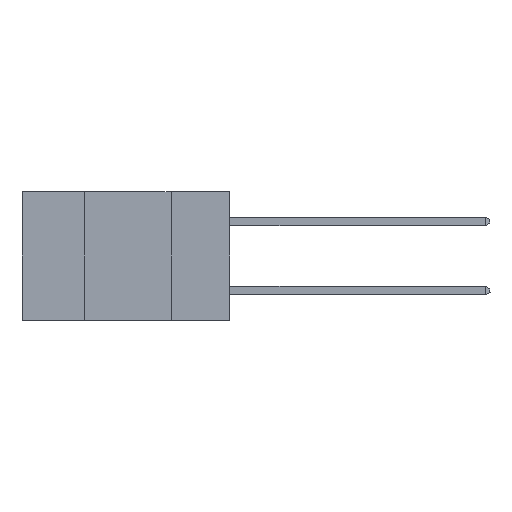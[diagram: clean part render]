
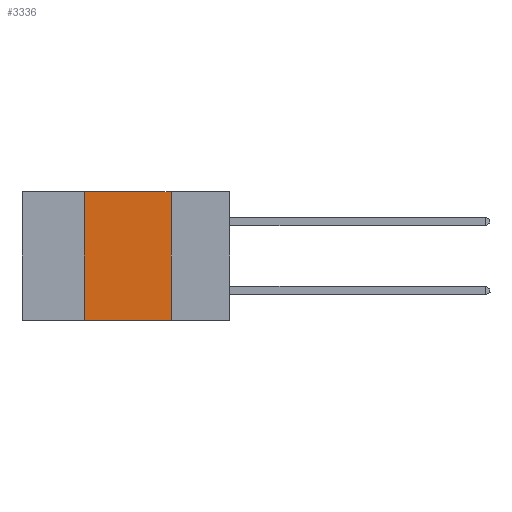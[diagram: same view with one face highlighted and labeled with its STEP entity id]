
A CAD part, left-side view. The second image highlights one B-rep face of the part: STEP entity #3336.
In plain terms, the highlighted planar face has unit normal (-1, 0, 0).
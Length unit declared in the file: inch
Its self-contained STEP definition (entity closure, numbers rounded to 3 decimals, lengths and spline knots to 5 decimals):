
#15 = EDGE_LOOP ( 'NONE', ( #10765, #5312, #13418, #7980 ) ) ;
#308 = FACE_OUTER_BOUND ( 'NONE', #15, .T. ) ;
#1269 = LINE ( 'NONE', #13963, #6182 ) ;
#1389 = CARTESIAN_POINT ( 'NONE',  ( 0., 0.6, 0. ) ) ;
#2230 = DIRECTION ( 'NONE',  ( 1., 0., 0. ) ) ;
#2913 = CARTESIAN_POINT ( 'NONE',  ( 0., 0.17, 0. ) ) ;
#3047 = CARTESIAN_POINT ( 'NONE',  ( 0., 0.17, 0. ) ) ;
#3236 = DIRECTION ( 'NONE',  ( 0., 0., 1. ) ) ;
#3336 = ADVANCED_FACE ( 'NONE', ( #308 ), #5546, .F. ) ;
#3437 = DIRECTION ( 'NONE',  ( 0., 0., -1. ) ) ;
#4242 = VERTEX_POINT ( 'NONE', #6245 ) ;
#4248 = EDGE_CURVE ( 'NONE', #11750, #12309, #8111, .T. ) ;
#4406 = LINE ( 'NONE', #2913, #5931 ) ;
#5312 = ORIENTED_EDGE ( 'NONE', *, *, #4248, .F. ) ;
#5546 = PLANE ( 'NONE',  #13192 ) ;
#5931 = VECTOR ( 'NONE', #11344, 39.37008 ) ;
#6182 = VECTOR ( 'NONE', #3236, 39.37008 ) ;
#6245 = CARTESIAN_POINT ( 'NONE',  ( 0., 0.17, -0.37 ) ) ;
#7114 = VECTOR ( 'NONE', #12608, 39.37008 ) ;
#7655 = CARTESIAN_POINT ( 'NONE',  ( 0., 0.42, -0.37 ) ) ;
#7980 = ORIENTED_EDGE ( 'NONE', *, *, #11260, .T. ) ;
#8111 = LINE ( 'NONE', #1389, #10176 ) ;
#8279 = LINE ( 'NONE', #12201, #7114 ) ;
#10176 = VECTOR ( 'NONE', #14512, 39.37008 ) ;
#10275 = CARTESIAN_POINT ( 'NONE',  ( 0., 0.42, 0. ) ) ;
#10432 = CARTESIAN_POINT ( 'NONE',  ( 0., 0.6, 0. ) ) ;
#10765 = ORIENTED_EDGE ( 'NONE', *, *, #13614, .F. ) ;
#11260 = EDGE_CURVE ( 'NONE', #12932, #4242, #8279, .T. ) ;
#11344 = DIRECTION ( 'NONE',  ( 0., 0., -1. ) ) ;
#11704 = EDGE_CURVE ( 'NONE', #12932, #11750, #1269, .T. ) ;
#11750 = VERTEX_POINT ( 'NONE', #10275 ) ;
#12201 = CARTESIAN_POINT ( 'NONE',  ( 0., 0.6, -0.37 ) ) ;
#12309 = VERTEX_POINT ( 'NONE', #3047 ) ;
#12608 = DIRECTION ( 'NONE',  ( 0., -1., 0. ) ) ;
#12932 = VERTEX_POINT ( 'NONE', #7655 ) ;
#13192 = AXIS2_PLACEMENT_3D ( 'NONE', #10432, #2230, #3437 ) ;
#13418 = ORIENTED_EDGE ( 'NONE', *, *, #11704, .F. ) ;
#13614 = EDGE_CURVE ( 'NONE', #12309, #4242, #4406, .T. ) ;
#13963 = CARTESIAN_POINT ( 'NONE',  ( 0., 0.42, 0. ) ) ;
#14512 = DIRECTION ( 'NONE',  ( 0., -1., 0. ) ) ;
